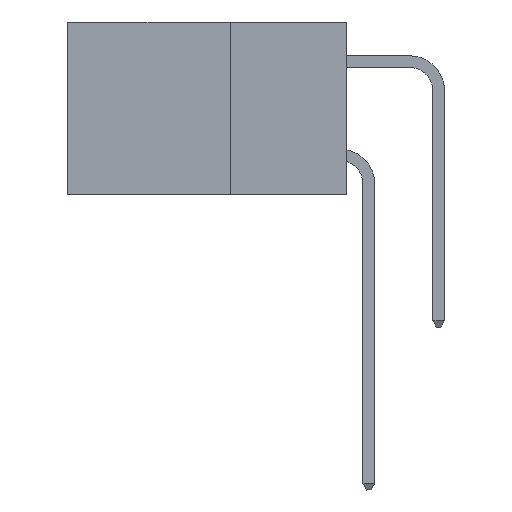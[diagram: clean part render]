
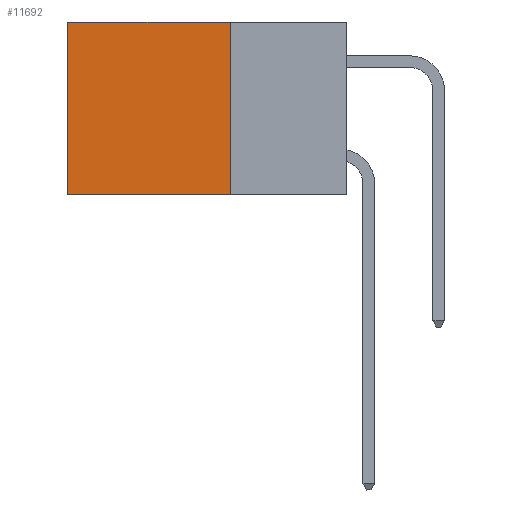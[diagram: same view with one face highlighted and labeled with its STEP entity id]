
A CAD part, left-side view. The second image highlights one B-rep face of the part: STEP entity #11692.
In plain terms, the highlighted planar face has unit normal (-1, 0, 0).
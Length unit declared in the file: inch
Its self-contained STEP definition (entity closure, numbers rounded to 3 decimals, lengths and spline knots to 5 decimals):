
#216 = CARTESIAN_POINT ( 'NONE',  ( 0.2875, 0.25, -0.37 ) ) ;
#396 = CARTESIAN_POINT ( 'NONE',  ( 0.2875, 0.6, -0.37 ) ) ;
#415 = PLANE ( 'NONE',  #26108 ) ;
#483 = DIRECTION ( 'NONE',  ( 0., 1., 0. ) ) ;
#1419 = EDGE_CURVE ( 'NONE', #18631, #15972, #1692, .T. ) ;
#1692 = LINE ( 'NONE', #9399, #5929 ) ;
#1881 = CARTESIAN_POINT ( 'NONE',  ( 0.2875, 0.6, 0. ) ) ;
#3362 = VERTEX_POINT ( 'NONE', #396 ) ;
#3686 = DIRECTION ( 'NONE',  ( 1., 0., 0. ) ) ;
#3872 = VECTOR ( 'NONE', #18747, 39.37008 ) ;
#5059 = ORIENTED_EDGE ( 'NONE', *, *, #1419, .F. ) ;
#5254 = ORIENTED_EDGE ( 'NONE', *, *, #18878, .F. ) ;
#5929 = VECTOR ( 'NONE', #13534, 39.37008 ) ;
#6841 = LINE ( 'NONE', #16616, #13256 ) ;
#7106 = CARTESIAN_POINT ( 'NONE',  ( 0.2875, 0.25, 0. ) ) ;
#8687 = CARTESIAN_POINT ( 'NONE',  ( 0.2875, 0.25, 0. ) ) ;
#9338 = LINE ( 'NONE', #8687, #3872 ) ;
#9399 = CARTESIAN_POINT ( 'NONE',  ( 0.2875, 0.25, 0. ) ) ;
#9912 = FACE_OUTER_BOUND ( 'NONE', #11560, .T. ) ;
#10029 = ORIENTED_EDGE ( 'NONE', *, *, #18765, .T. ) ;
#10232 = DIRECTION ( 'NONE',  ( 0., 0., -1. ) ) ;
#11560 = EDGE_LOOP ( 'NONE', ( #10029, #5254, #5059, #13823 ) ) ;
#11692 = ADVANCED_FACE ( 'NONE', ( #9912 ), #415, .F. ) ;
#13256 = VECTOR ( 'NONE', #483, 39.37008 ) ;
#13534 = DIRECTION ( 'NONE',  ( 0., 0., -1. ) ) ;
#13823 = ORIENTED_EDGE ( 'NONE', *, *, #14416, .T. ) ;
#14416 = EDGE_CURVE ( 'NONE', #18631, #20775, #9338, .T. ) ;
#15972 = VERTEX_POINT ( 'NONE', #216 ) ;
#16616 = CARTESIAN_POINT ( 'NONE',  ( 0.2875, 0.25, -0.37 ) ) ;
#18412 = LINE ( 'NONE', #22778, #21329 ) ;
#18631 = VERTEX_POINT ( 'NONE', #20035 ) ;
#18747 = DIRECTION ( 'NONE',  ( 0., 1., 0. ) ) ;
#18765 = EDGE_CURVE ( 'NONE', #20775, #3362, #18412, .T. ) ;
#18878 = EDGE_CURVE ( 'NONE', #15972, #3362, #6841, .T. ) ;
#20035 = CARTESIAN_POINT ( 'NONE',  ( 0.2875, 0.25, 0. ) ) ;
#20135 = DIRECTION ( 'NONE',  ( 0., 0., -1. ) ) ;
#20775 = VERTEX_POINT ( 'NONE', #1881 ) ;
#21329 = VECTOR ( 'NONE', #10232, 39.37008 ) ;
#22778 = CARTESIAN_POINT ( 'NONE',  ( 0.2875, 0.6, 0. ) ) ;
#26108 = AXIS2_PLACEMENT_3D ( 'NONE', #7106, #3686, #20135 ) ;
